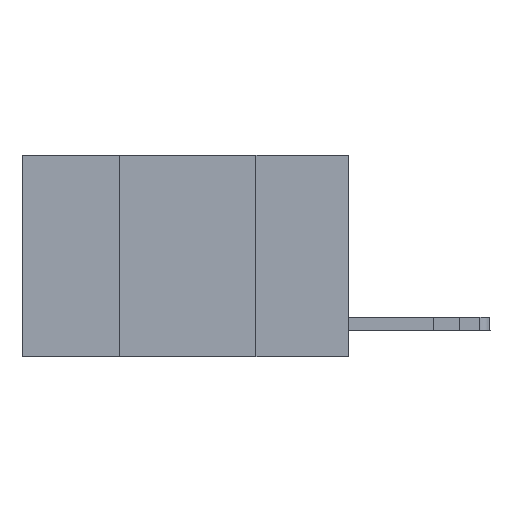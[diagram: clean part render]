
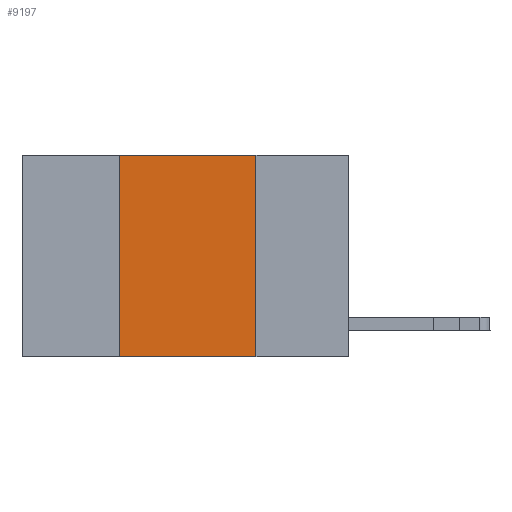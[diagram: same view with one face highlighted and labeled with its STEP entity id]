
A CAD part, left-side view. The second image highlights one B-rep face of the part: STEP entity #9197.
In plain terms, the highlighted planar face has unit normal (-1, 0, 0).
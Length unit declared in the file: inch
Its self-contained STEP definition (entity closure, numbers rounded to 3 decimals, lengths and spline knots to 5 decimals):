
#339 = ORIENTED_EDGE ( 'NONE', *, *, #10011, .T. ) ;
#396 = LINE ( 'NONE', #6668, #9477 ) ;
#651 = LINE ( 'NONE', #12533, #5362 ) ;
#876 = CARTESIAN_POINT ( 'NONE',  ( 0., 0.6, 0. ) ) ;
#1289 = DIRECTION ( 'NONE',  ( 0., -1., 0. ) ) ;
#1323 = AXIS2_PLACEMENT_3D ( 'NONE', #876, #8824, #2053 ) ;
#1807 = VECTOR ( 'NONE', #11903, 39.37008 ) ;
#1978 = FACE_OUTER_BOUND ( 'NONE', #4851, .T. ) ;
#1988 = VERTEX_POINT ( 'NONE', #13106 ) ;
#2053 = DIRECTION ( 'NONE',  ( 0., 0., -1. ) ) ;
#3279 = EDGE_CURVE ( 'NONE', #7884, #1988, #6371, .T. ) ;
#3366 = CARTESIAN_POINT ( 'NONE',  ( 0., 0.6, 0. ) ) ;
#3514 = DIRECTION ( 'NONE',  ( 0., -1., 0. ) ) ;
#4007 = ORIENTED_EDGE ( 'NONE', *, *, #9026, .F. ) ;
#4235 = VERTEX_POINT ( 'NONE', #5841 ) ;
#4851 = EDGE_LOOP ( 'NONE', ( #4007, #9083, #5531, #339 ) ) ;
#5362 = VECTOR ( 'NONE', #1289, 39.37008 ) ;
#5526 = EDGE_CURVE ( 'NONE', #7007, #7884, #396, .T. ) ;
#5531 = ORIENTED_EDGE ( 'NONE', *, *, #5526, .F. ) ;
#5684 = VECTOR ( 'NONE', #3514, 39.37008 ) ;
#5841 = CARTESIAN_POINT ( 'NONE',  ( 0., 0.17, -0.37 ) ) ;
#6371 = LINE ( 'NONE', #3366, #5684 ) ;
#6668 = CARTESIAN_POINT ( 'NONE',  ( 0., 0.42, 0. ) ) ;
#7007 = VERTEX_POINT ( 'NONE', #8144 ) ;
#7500 = LINE ( 'NONE', #10781, #1807 ) ;
#7884 = VERTEX_POINT ( 'NONE', #12115 ) ;
#8144 = CARTESIAN_POINT ( 'NONE',  ( 0., 0.42, -0.37 ) ) ;
#8824 = DIRECTION ( 'NONE',  ( 1., 0., 0. ) ) ;
#8908 = DIRECTION ( 'NONE',  ( 0., 0., 1. ) ) ;
#9026 = EDGE_CURVE ( 'NONE', #1988, #4235, #7500, .T. ) ;
#9083 = ORIENTED_EDGE ( 'NONE', *, *, #3279, .F. ) ;
#9197 = ADVANCED_FACE ( 'NONE', ( #1978 ), #13177, .F. ) ;
#9477 = VECTOR ( 'NONE', #8908, 39.37008 ) ;
#10011 = EDGE_CURVE ( 'NONE', #7007, #4235, #651, .T. ) ;
#10781 = CARTESIAN_POINT ( 'NONE',  ( 0., 0.17, 0. ) ) ;
#11903 = DIRECTION ( 'NONE',  ( 0., 0., -1. ) ) ;
#12115 = CARTESIAN_POINT ( 'NONE',  ( 0., 0.42, 0. ) ) ;
#12533 = CARTESIAN_POINT ( 'NONE',  ( 0., 0.6, -0.37 ) ) ;
#13106 = CARTESIAN_POINT ( 'NONE',  ( 0., 0.17, 0. ) ) ;
#13177 = PLANE ( 'NONE',  #1323 ) ;
